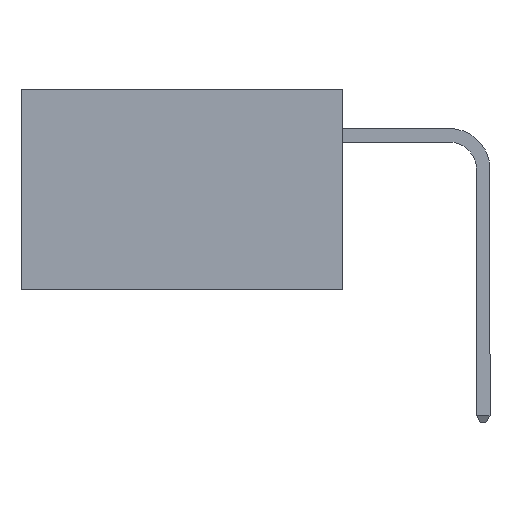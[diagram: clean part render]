
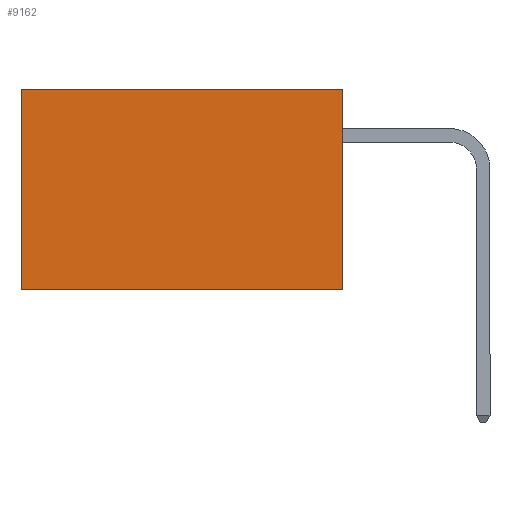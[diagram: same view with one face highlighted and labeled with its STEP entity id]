
A CAD part, left-side view. The second image highlights one B-rep face of the part: STEP entity #9162.
In plain terms, the highlighted planar face has unit normal (-1, 0, 0).
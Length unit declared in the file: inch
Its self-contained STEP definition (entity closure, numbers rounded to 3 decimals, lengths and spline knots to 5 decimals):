
#19 = VERTEX_POINT ( 'NONE', #1226 ) ;
#336 = EDGE_CURVE ( 'NONE', #19, #1436, #4340, .T. ) ;
#341 = LINE ( 'NONE', #390, #6197 ) ;
#390 = CARTESIAN_POINT ( 'NONE',  ( 0.277, 0., 0. ) ) ;
#416 = EDGE_CURVE ( 'NONE', #821, #5728, #2017, .T. ) ;
#603 = DIRECTION ( 'NONE',  ( 1., 0., 0. ) ) ;
#720 = FACE_OUTER_BOUND ( 'NONE', #6139, .T. ) ;
#821 = VERTEX_POINT ( 'NONE', #3175 ) ;
#970 = ORIENTED_EDGE ( 'NONE', *, *, #336, .T. ) ;
#1226 = CARTESIAN_POINT ( 'NONE',  ( 0.277, 0.59, 0. ) ) ;
#1436 = VERTEX_POINT ( 'NONE', #5482 ) ;
#1580 = CARTESIAN_POINT ( 'NONE',  ( 0.277, 0., -0.37 ) ) ;
#1601 = VECTOR ( 'NONE', #4449, 39.37008 ) ;
#2017 = LINE ( 'NONE', #2798, #5383 ) ;
#2707 = DIRECTION ( 'NONE',  ( 0., 0., -1. ) ) ;
#2798 = CARTESIAN_POINT ( 'NONE',  ( 0.277, 0., -0.37 ) ) ;
#3175 = CARTESIAN_POINT ( 'NONE',  ( 0.277, 0., 0. ) ) ;
#3879 = CARTESIAN_POINT ( 'NONE',  ( 0.277, 0.59, -0.37 ) ) ;
#4166 = LINE ( 'NONE', #1580, #1601 ) ;
#4340 = LINE ( 'NONE', #3879, #7652 ) ;
#4449 = DIRECTION ( 'NONE',  ( 0., 1., 0. ) ) ;
#4797 = ORIENTED_EDGE ( 'NONE', *, *, #8054, .F. ) ;
#4996 = CARTESIAN_POINT ( 'NONE',  ( 0.277, 0., -0.37 ) ) ;
#5383 = VECTOR ( 'NONE', #2707, 39.37008 ) ;
#5482 = CARTESIAN_POINT ( 'NONE',  ( 0.277, 0.59, -0.37 ) ) ;
#5703 = DIRECTION ( 'NONE',  ( 0., 0., -1. ) ) ;
#5728 = VERTEX_POINT ( 'NONE', #6510 ) ;
#6139 = EDGE_LOOP ( 'NONE', ( #970, #4797, #7866, #7095 ) ) ;
#6197 = VECTOR ( 'NONE', #6930, 39.37008 ) ;
#6510 = CARTESIAN_POINT ( 'NONE',  ( 0.277, 0., -0.37 ) ) ;
#6930 = DIRECTION ( 'NONE',  ( 0., 1., 0. ) ) ;
#7095 = ORIENTED_EDGE ( 'NONE', *, *, #8987, .T. ) ;
#7652 = VECTOR ( 'NONE', #8051, 39.37008 ) ;
#7866 = ORIENTED_EDGE ( 'NONE', *, *, #416, .F. ) ;
#8051 = DIRECTION ( 'NONE',  ( 0., 0., -1. ) ) ;
#8054 = EDGE_CURVE ( 'NONE', #5728, #1436, #4166, .T. ) ;
#8164 = AXIS2_PLACEMENT_3D ( 'NONE', #4996, #603, #5703 ) ;
#8987 = EDGE_CURVE ( 'NONE', #821, #19, #341, .T. ) ;
#9123 = PLANE ( 'NONE',  #8164 ) ;
#9162 = ADVANCED_FACE ( 'NONE', ( #720 ), #9123, .F. ) ;
